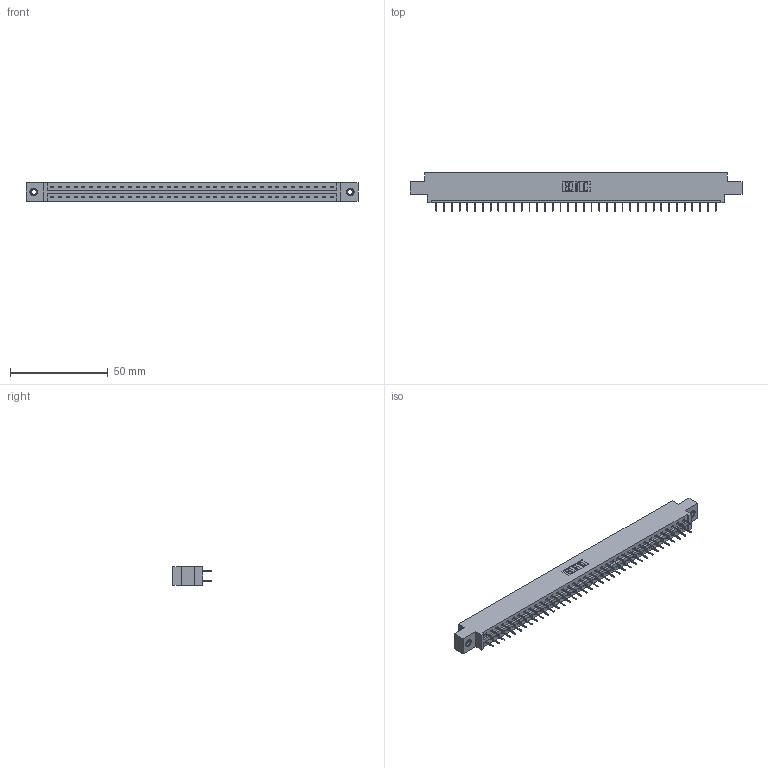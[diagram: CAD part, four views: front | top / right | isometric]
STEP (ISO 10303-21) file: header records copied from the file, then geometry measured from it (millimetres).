
FILE_DESCRIPTION (( 'STEP AP203' ), '1' );
FILE_NAME ('337-074-524-807.STEP', '2019-10-15T12:23:56', ( '' ), ( '' ), 'SwSTEP 2.0', 'SolidWorks 2016', '' );
FILE_SCHEMA (( 'CONFIG_CONTROL_DESIGN' ));
Length unit declared in the file: inch
Products named in the file (4): 337 Part_0.170 Offset - 0.156 Dia-TI; 345-250-001_345-250-005-103; 345-292-001_345-293-124; 337-074-524-807
Assembly tree (77 placements, depth 2):
  337-074-524-807
    337 Part_0.170 Offset - 0.156 Dia-TI
    345-292-001_345-293-124  x74
    345-250-001_345-250-005-103  x2
Bounding box: 169.62 x 19.69 x 9.4 mm (x, y, z)
Volume: 17566.5 mm3; surface area: 19607.3 mm2
Topology: 77 solids, 77 shells, 4470 faces, 12669 edges, 8142 vertices
Faces by surface type: plane 3362, cylinder 1092, cone 12, torus 4
Entity records: 30726 total; most frequent: CARTESIAN_POINT 5161, ORIENTED_EDGE 5090, DIRECTION 4431, EDGE_CURVE 2545, VECTOR 2401, LINE 2401, VERTEX_POINT 1688, AXIS2_PLACEMENT_3D 1015
